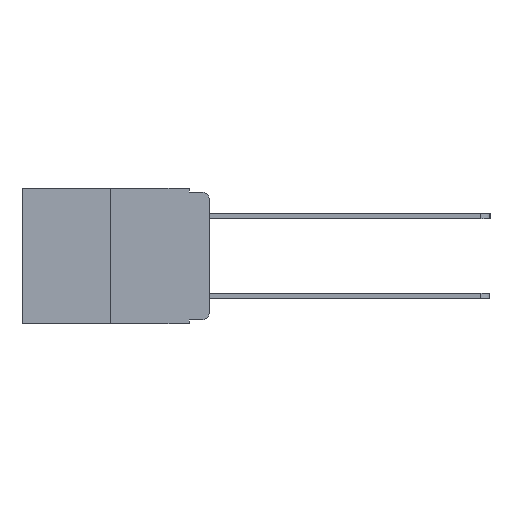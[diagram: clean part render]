
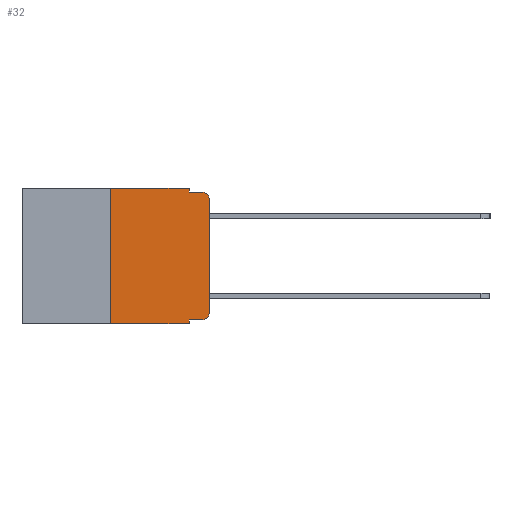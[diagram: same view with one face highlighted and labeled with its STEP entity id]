
A CAD part, left-side view. The second image highlights one B-rep face of the part: STEP entity #32.
In plain terms, the highlighted planar face has unit normal (-1, 0, 0).
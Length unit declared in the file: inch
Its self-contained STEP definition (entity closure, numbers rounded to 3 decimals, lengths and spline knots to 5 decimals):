
#32 = ADVANCED_FACE ( 'NONE', ( #10451 ), #2615, .F. ) ;
#33 = CARTESIAN_POINT ( 'NONE',  ( 0., 0.02, -0.01 ) ) ;
#35 = CARTESIAN_POINT ( 'NONE',  ( 0., 0.02, -0.03 ) ) ;
#42 = ORIENTED_EDGE ( 'NONE', *, *, #2429, .F. ) ;
#242 = DIRECTION ( 'NONE',  ( 0., -1., 0. ) ) ;
#323 = DIRECTION ( 'NONE',  ( -1., 0., 0. ) ) ;
#352 = VECTOR ( 'NONE', #2966, 39.37008 ) ;
#595 = EDGE_CURVE ( 'NONE', #2735, #13295, #16499, .T. ) ;
#719 = EDGE_CURVE ( 'NONE', #6345, #2735, #4649, .T. ) ;
#792 = VERTEX_POINT ( 'NONE', #5715 ) ;
#1316 = VECTOR ( 'NONE', #13473, 39.37008 ) ;
#1489 = VERTEX_POINT ( 'NONE', #13039 ) ;
#1534 = VERTEX_POINT ( 'NONE', #3205 ) ;
#1626 = DIRECTION ( 'NONE',  ( 0., 0., -1. ) ) ;
#1961 = CARTESIAN_POINT ( 'NONE',  ( 0., 0.051, -0.01 ) ) ;
#2095 = EDGE_CURVE ( 'NONE', #792, #1534, #17003, .T. ) ;
#2202 = CARTESIAN_POINT ( 'NONE',  ( 0., 0.473, 0. ) ) ;
#2227 = VECTOR ( 'NONE', #7987, 39.37008 ) ;
#2429 = EDGE_CURVE ( 'NONE', #12854, #9633, #3187, .T. ) ;
#2615 = PLANE ( 'NONE',  #13956 ) ;
#2735 = VERTEX_POINT ( 'NONE', #4476 ) ;
#2892 = CARTESIAN_POINT ( 'NONE',  ( 0., 0.051, 0. ) ) ;
#2966 = DIRECTION ( 'NONE',  ( 0., 0., 1. ) ) ;
#2968 = VECTOR ( 'NONE', #242, 39.37008 ) ;
#3187 = LINE ( 'NONE', #15134, #10246 ) ;
#3205 = CARTESIAN_POINT ( 'NONE',  ( 0., 0.051, 0. ) ) ;
#3755 = ORIENTED_EDGE ( 'NONE', *, *, #4525, .F. ) ;
#4058 = DIRECTION ( 'NONE',  ( 0., 0., -1. ) ) ;
#4103 = EDGE_LOOP ( 'NONE', ( #15665, #6377, #13333, #7279, #10642, #3755, #14041, #42, #4710, #11712 ) ) ;
#4135 = LINE ( 'NONE', #6645, #11280 ) ;
#4476 = CARTESIAN_POINT ( 'NONE',  ( 0., 0., -0.313 ) ) ;
#4525 = EDGE_CURVE ( 'NONE', #1489, #792, #7993, .T. ) ;
#4649 = CIRCLE ( 'NONE', #10807, 0.02 ) ;
#4710 = ORIENTED_EDGE ( 'NONE', *, *, #9598, .T. ) ;
#4773 = DIRECTION ( 'NONE',  ( 0., -1., 0. ) ) ;
#4787 = CARTESIAN_POINT ( 'NONE',  ( 0., 0.473, 0. ) ) ;
#4914 = CARTESIAN_POINT ( 'NONE',  ( 0., 0.02, -0.333 ) ) ;
#5477 = LINE ( 'NONE', #2892, #1316 ) ;
#5553 = EDGE_CURVE ( 'NONE', #1534, #15839, #5477, .T. ) ;
#5715 = CARTESIAN_POINT ( 'NONE',  ( 0., 0.25, 0. ) ) ;
#6345 = VERTEX_POINT ( 'NONE', #4914 ) ;
#6377 = ORIENTED_EDGE ( 'NONE', *, *, #10872, .T. ) ;
#6645 = CARTESIAN_POINT ( 'NONE',  ( 0., 0.051, -0.333 ) ) ;
#6689 = CARTESIAN_POINT ( 'NONE',  ( 0., 0.051, -0.01 ) ) ;
#6763 = EDGE_CURVE ( 'NONE', #1489, #9633, #13151, .T. ) ;
#7279 = ORIENTED_EDGE ( 'NONE', *, *, #5553, .F. ) ;
#7369 = CARTESIAN_POINT ( 'NONE',  ( 0., 0.02, -0.313 ) ) ;
#7452 = VECTOR ( 'NONE', #7643, 39.37008 ) ;
#7508 = EDGE_CURVE ( 'NONE', #15839, #9285, #15644, .T. ) ;
#7643 = DIRECTION ( 'NONE',  ( 0., 0., 1. ) ) ;
#7816 = CIRCLE ( 'NONE', #15735, 0.02 ) ;
#7987 = DIRECTION ( 'NONE',  ( 0., -1., 0. ) ) ;
#7993 = LINE ( 'NONE', #13531, #352 ) ;
#9285 = VERTEX_POINT ( 'NONE', #33 ) ;
#9598 = EDGE_CURVE ( 'NONE', #12854, #6345, #4135, .T. ) ;
#9633 = VERTEX_POINT ( 'NONE', #15132 ) ;
#10236 = DIRECTION ( 'NONE',  ( -1., 0., 0. ) ) ;
#10246 = VECTOR ( 'NONE', #15299, 39.37008 ) ;
#10377 = CARTESIAN_POINT ( 'NONE',  ( 0., 0.473, -0.343 ) ) ;
#10451 = FACE_OUTER_BOUND ( 'NONE', #4103, .T. ) ;
#10642 = ORIENTED_EDGE ( 'NONE', *, *, #2095, .F. ) ;
#10807 = AXIS2_PLACEMENT_3D ( 'NONE', #7369, #323, #13984 ) ;
#10872 = EDGE_CURVE ( 'NONE', #13295, #9285, #7816, .T. ) ;
#10979 = VECTOR ( 'NONE', #4773, 39.37008 ) ;
#11280 = VECTOR ( 'NONE', #16227, 39.37008 ) ;
#11712 = ORIENTED_EDGE ( 'NONE', *, *, #719, .T. ) ;
#12854 = VERTEX_POINT ( 'NONE', #16774 ) ;
#13039 = CARTESIAN_POINT ( 'NONE',  ( 0., 0.25, -0.343 ) ) ;
#13151 = LINE ( 'NONE', #10377, #2968 ) ;
#13248 = CARTESIAN_POINT ( 'NONE',  ( 0., 0., 0. ) ) ;
#13295 = VERTEX_POINT ( 'NONE', #14991 ) ;
#13333 = ORIENTED_EDGE ( 'NONE', *, *, #7508, .F. ) ;
#13473 = DIRECTION ( 'NONE',  ( 0., 0., -1. ) ) ;
#13531 = CARTESIAN_POINT ( 'NONE',  ( 0., 0.25, 0. ) ) ;
#13956 = AXIS2_PLACEMENT_3D ( 'NONE', #2202, #15006, #4058 ) ;
#13984 = DIRECTION ( 'NONE',  ( 0., 0., -1. ) ) ;
#14041 = ORIENTED_EDGE ( 'NONE', *, *, #6763, .T. ) ;
#14991 = CARTESIAN_POINT ( 'NONE',  ( 0., 0., -0.03 ) ) ;
#15006 = DIRECTION ( 'NONE',  ( 1., 0., 0. ) ) ;
#15132 = CARTESIAN_POINT ( 'NONE',  ( 0., 0.051, -0.343 ) ) ;
#15134 = CARTESIAN_POINT ( 'NONE',  ( 0., 0.051, 0. ) ) ;
#15299 = DIRECTION ( 'NONE',  ( 0., 0., -1. ) ) ;
#15644 = LINE ( 'NONE', #1961, #2227 ) ;
#15665 = ORIENTED_EDGE ( 'NONE', *, *, #595, .T. ) ;
#15735 = AXIS2_PLACEMENT_3D ( 'NONE', #35, #10236, #1626 ) ;
#15839 = VERTEX_POINT ( 'NONE', #6689 ) ;
#16227 = DIRECTION ( 'NONE',  ( 0., -1., 0. ) ) ;
#16499 = LINE ( 'NONE', #13248, #7452 ) ;
#16774 = CARTESIAN_POINT ( 'NONE',  ( 0., 0.051, -0.333 ) ) ;
#17003 = LINE ( 'NONE', #4787, #10979 ) ;
